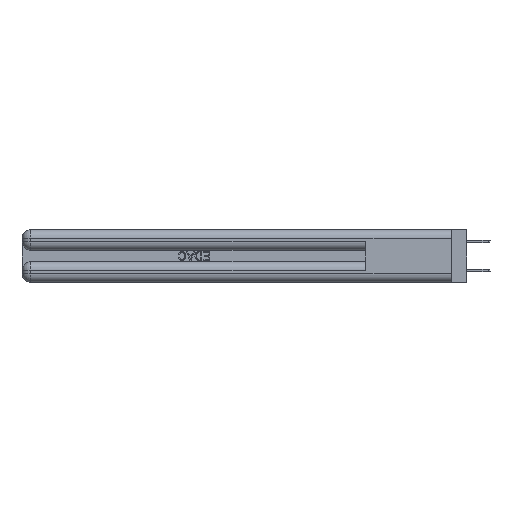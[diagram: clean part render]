
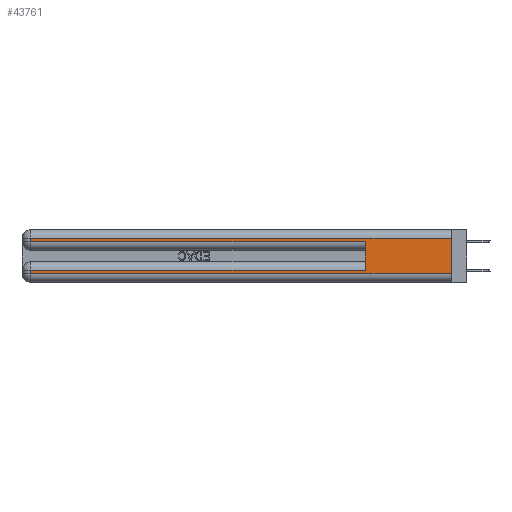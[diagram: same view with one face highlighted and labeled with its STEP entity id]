
A CAD part, left-side view. The second image highlights one B-rep face of the part: STEP entity #43761.
In plain terms, the highlighted planar face has unit normal (-1, 0, 0).
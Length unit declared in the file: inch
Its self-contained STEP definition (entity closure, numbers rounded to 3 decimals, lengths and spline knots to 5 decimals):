
#87 = VECTOR ( 'NONE', #33781, 39.37008 ) ;
#394 = CARTESIAN_POINT ( 'NONE',  ( 0., 2.94, 0.37 ) ) ;
#420 = EDGE_CURVE ( 'NONE', #29288, #40109, #36532, .T. ) ;
#2046 = AXIS2_PLACEMENT_3D ( 'NONE', #14969, #18453, #42026 ) ;
#3738 = VECTOR ( 'NONE', #30619, 39.37008 ) ;
#4319 = ORIENTED_EDGE ( 'NONE', *, *, #36791, .T. ) ;
#4421 = ORIENTED_EDGE ( 'NONE', *, *, #30899, .T. ) ;
#4913 = CARTESIAN_POINT ( 'NONE',  ( 0., 0., 0.31 ) ) ;
#5648 = CARTESIAN_POINT ( 'NONE',  ( 0., 2.94, 0.285 ) ) ;
#6963 = CARTESIAN_POINT ( 'NONE',  ( 0., 0., 0.06 ) ) ;
#7331 = CARTESIAN_POINT ( 'NONE',  ( 0., 2.94, 0.31 ) ) ;
#7771 = LINE ( 'NONE', #9596, #35006 ) ;
#7992 = PLANE ( 'NONE',  #2046 ) ;
#8374 = VECTOR ( 'NONE', #9200, 39.37008 ) ;
#8615 = ORIENTED_EDGE ( 'NONE', *, *, #25901, .T. ) ;
#8909 = ORIENTED_EDGE ( 'NONE', *, *, #12409, .T. ) ;
#9200 = DIRECTION ( 'NONE',  ( 0., 0., 1. ) ) ;
#9464 = LINE ( 'NONE', #16161, #8374 ) ;
#9596 = CARTESIAN_POINT ( 'NONE',  ( 0., 0., 0.31 ) ) ;
#9900 = CARTESIAN_POINT ( 'NONE',  ( 0., 0., 0.085 ) ) ;
#10078 = ORIENTED_EDGE ( 'NONE', *, *, #420, .T. ) ;
#10140 = CARTESIAN_POINT ( 'NONE',  ( 0., 0., 0.285 ) ) ;
#11179 = VERTEX_POINT ( 'NONE', #18296 ) ;
#11542 = ORIENTED_EDGE ( 'NONE', *, *, #30140, .F. ) ;
#11725 = ORIENTED_EDGE ( 'NONE', *, *, #18881, .T. ) ;
#11751 = VERTEX_POINT ( 'NONE', #7331 ) ;
#12409 = EDGE_CURVE ( 'NONE', #40109, #13022, #22539, .T. ) ;
#13022 = VERTEX_POINT ( 'NONE', #34845 ) ;
#13246 = VERTEX_POINT ( 'NONE', #5648 ) ;
#13379 = VECTOR ( 'NONE', #28107, 39.37008 ) ;
#13975 = CARTESIAN_POINT ( 'NONE',  ( 0., 2.94, 0.37 ) ) ;
#14969 = CARTESIAN_POINT ( 'NONE',  ( 0., 0., 0.37 ) ) ;
#16161 = CARTESIAN_POINT ( 'NONE',  ( 0., 0.6, 0.145 ) ) ;
#18296 = CARTESIAN_POINT ( 'NONE',  ( 0., 0., 0.06 ) ) ;
#18453 = DIRECTION ( 'NONE',  ( 1., 0., 0. ) ) ;
#18881 = EDGE_CURVE ( 'NONE', #13246, #43704, #29046, .T. ) ;
#19469 = VECTOR ( 'NONE', #20863, 39.37008 ) ;
#20863 = DIRECTION ( 'NONE',  ( 0., -1., 0. ) ) ;
#21287 = CARTESIAN_POINT ( 'NONE',  ( 0., 0.6, 0.285 ) ) ;
#21989 = FACE_OUTER_BOUND ( 'NONE', #31622, .T. ) ;
#22077 = EDGE_CURVE ( 'NONE', #26169, #11179, #22937, .T. ) ;
#22539 = LINE ( 'NONE', #394, #13379 ) ;
#22937 = LINE ( 'NONE', #37093, #30887 ) ;
#25901 = EDGE_CURVE ( 'NONE', #13022, #11179, #30595, .T. ) ;
#26169 = VERTEX_POINT ( 'NONE', #4913 ) ;
#28107 = DIRECTION ( 'NONE',  ( 0., 0., -1. ) ) ;
#29046 = LINE ( 'NONE', #10140, #3738 ) ;
#29288 = VERTEX_POINT ( 'NONE', #34769 ) ;
#30140 = EDGE_CURVE ( 'NONE', #29288, #43704, #9464, .T. ) ;
#30595 = LINE ( 'NONE', #6963, #19469 ) ;
#30619 = DIRECTION ( 'NONE',  ( 0., -1., 0. ) ) ;
#30887 = VECTOR ( 'NONE', #40457, 39.37008 ) ;
#30899 = EDGE_CURVE ( 'NONE', #26169, #11751, #7771, .T. ) ;
#31622 = EDGE_LOOP ( 'NONE', ( #39849, #4421, #4319, #11725, #11542, #10078, #8909, #8615 ) ) ;
#33472 = DIRECTION ( 'NONE',  ( 0., 1., 0. ) ) ;
#33781 = DIRECTION ( 'NONE',  ( 0., 1., 0. ) ) ;
#33812 = CARTESIAN_POINT ( 'NONE',  ( 0., 2.94, 0.085 ) ) ;
#34072 = VECTOR ( 'NONE', #34365, 39.37008 ) ;
#34365 = DIRECTION ( 'NONE',  ( 0., 0., -1. ) ) ;
#34769 = CARTESIAN_POINT ( 'NONE',  ( 0., 0.6, 0.085 ) ) ;
#34845 = CARTESIAN_POINT ( 'NONE',  ( 0., 2.94, 0.06 ) ) ;
#35006 = VECTOR ( 'NONE', #33472, 39.37008 ) ;
#35113 = LINE ( 'NONE', #13975, #34072 ) ;
#36532 = LINE ( 'NONE', #9900, #87 ) ;
#36791 = EDGE_CURVE ( 'NONE', #11751, #13246, #35113, .T. ) ;
#37093 = CARTESIAN_POINT ( 'NONE',  ( 0., 0., 0.37 ) ) ;
#39849 = ORIENTED_EDGE ( 'NONE', *, *, #22077, .F. ) ;
#40109 = VERTEX_POINT ( 'NONE', #33812 ) ;
#40457 = DIRECTION ( 'NONE',  ( 0., 0., -1. ) ) ;
#42026 = DIRECTION ( 'NONE',  ( 0., 0., -1. ) ) ;
#43704 = VERTEX_POINT ( 'NONE', #21287 ) ;
#43761 = ADVANCED_FACE ( 'NONE', ( #21989 ), #7992, .F. ) ;
